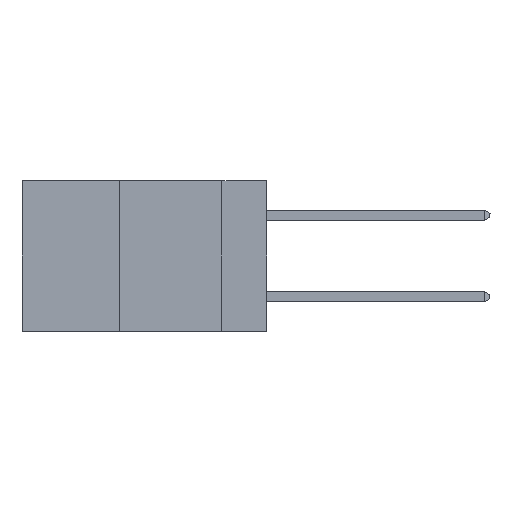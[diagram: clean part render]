
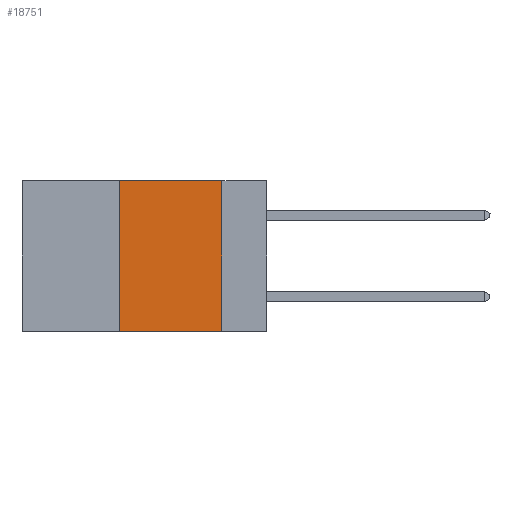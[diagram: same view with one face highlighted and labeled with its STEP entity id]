
A CAD part, left-side view. The second image highlights one B-rep face of the part: STEP entity #18751.
In plain terms, the highlighted planar face has unit normal (-1, 0, 0).
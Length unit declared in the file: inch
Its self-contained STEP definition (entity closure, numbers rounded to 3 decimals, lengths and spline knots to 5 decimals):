
#649 = EDGE_CURVE ( 'NONE', #8002, #14913, #12292, .T. ) ;
#2699 = ORIENTED_EDGE ( 'NONE', *, *, #649, .F. ) ;
#3719 = ORIENTED_EDGE ( 'NONE', *, *, #8909, .T. ) ;
#4108 = PLANE ( 'NONE',  #20224 ) ;
#4297 = CARTESIAN_POINT ( 'NONE',  ( 0., 0.11, -0.37 ) ) ;
#5145 = CARTESIAN_POINT ( 'NONE',  ( 0., 0.11, 0. ) ) ;
#5499 = VECTOR ( 'NONE', #26944, 39.37008 ) ;
#5973 = DIRECTION ( 'NONE',  ( 0., 0., 1. ) ) ;
#6609 = EDGE_LOOP ( 'NONE', ( #7413, #7142, #2699, #3719 ) ) ;
#7142 = ORIENTED_EDGE ( 'NONE', *, *, #17628, .F. ) ;
#7286 = DIRECTION ( 'NONE',  ( 0., 0., -1. ) ) ;
#7413 = ORIENTED_EDGE ( 'NONE', *, *, #9792, .F. ) ;
#8002 = VERTEX_POINT ( 'NONE', #10092 ) ;
#8909 = EDGE_CURVE ( 'NONE', #8002, #21619, #9884, .T. ) ;
#9120 = VECTOR ( 'NONE', #7286, 39.37008 ) ;
#9792 = EDGE_CURVE ( 'NONE', #10195, #21619, #24803, .T. ) ;
#9884 = LINE ( 'NONE', #15908, #5499 ) ;
#10092 = CARTESIAN_POINT ( 'NONE',  ( 0., 0.36, -0.37 ) ) ;
#10195 = VERTEX_POINT ( 'NONE', #22520 ) ;
#12292 = LINE ( 'NONE', #21207, #14813 ) ;
#12305 = DIRECTION ( 'NONE',  ( 0., 0., -1. ) ) ;
#12844 = VECTOR ( 'NONE', #17684, 39.37008 ) ;
#14813 = VECTOR ( 'NONE', #5973, 39.37008 ) ;
#14880 = FACE_OUTER_BOUND ( 'NONE', #6609, .T. ) ;
#14913 = VERTEX_POINT ( 'NONE', #17539 ) ;
#15535 = CARTESIAN_POINT ( 'NONE',  ( 0., 0.6, 0. ) ) ;
#15908 = CARTESIAN_POINT ( 'NONE',  ( 0., 0.6, -0.37 ) ) ;
#17539 = CARTESIAN_POINT ( 'NONE',  ( 0., 0.36, 0. ) ) ;
#17628 = EDGE_CURVE ( 'NONE', #14913, #10195, #26730, .T. ) ;
#17684 = DIRECTION ( 'NONE',  ( 0., -1., 0. ) ) ;
#18751 = ADVANCED_FACE ( 'NONE', ( #14880 ), #4108, .F. ) ;
#20224 = AXIS2_PLACEMENT_3D ( 'NONE', #23770, #27651, #12305 ) ;
#21207 = CARTESIAN_POINT ( 'NONE',  ( 0., 0.36, 0. ) ) ;
#21619 = VERTEX_POINT ( 'NONE', #4297 ) ;
#22520 = CARTESIAN_POINT ( 'NONE',  ( 0., 0.11, 0. ) ) ;
#23770 = CARTESIAN_POINT ( 'NONE',  ( 0., 0.6, 0. ) ) ;
#24803 = LINE ( 'NONE', #5145, #9120 ) ;
#26730 = LINE ( 'NONE', #15535, #12844 ) ;
#26944 = DIRECTION ( 'NONE',  ( 0., -1., 0. ) ) ;
#27651 = DIRECTION ( 'NONE',  ( 1., 0., 0. ) ) ;
